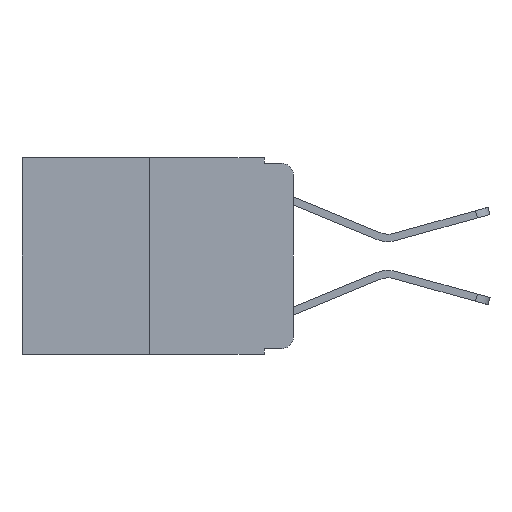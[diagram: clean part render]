
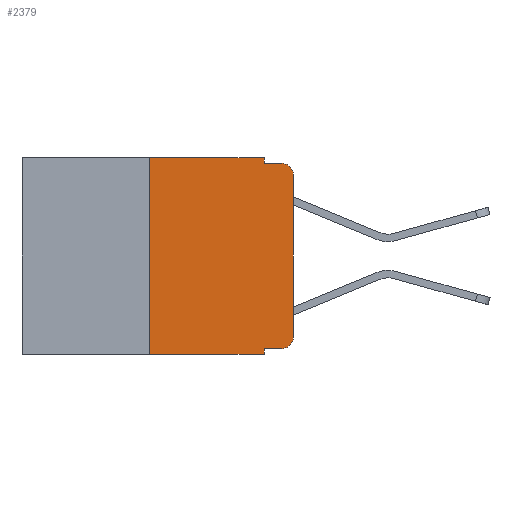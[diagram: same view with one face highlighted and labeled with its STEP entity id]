
A CAD part, left-side view. The second image highlights one B-rep face of the part: STEP entity #2379.
In plain terms, the highlighted planar face has unit normal (-1, 0, 0).
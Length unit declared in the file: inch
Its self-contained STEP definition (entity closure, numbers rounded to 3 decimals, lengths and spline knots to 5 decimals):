
#25 = CARTESIAN_POINT ( 'NONE',  ( 0., 0.473, -0.343 ) ) ;
#545 = EDGE_CURVE ( 'NONE', #8160, #2380, #8892, .T. ) ;
#1359 = ORIENTED_EDGE ( 'NONE', *, *, #10908, .F. ) ;
#1420 = DIRECTION ( 'NONE',  ( 0., -1., 0. ) ) ;
#1540 = CARTESIAN_POINT ( 'NONE',  ( 0., 0.02, -0.313 ) ) ;
#1792 = LINE ( 'NONE', #3881, #6658 ) ;
#1939 = ORIENTED_EDGE ( 'NONE', *, *, #9270, .T. ) ;
#1943 = CARTESIAN_POINT ( 'NONE',  ( 0., 0.051, -0.333 ) ) ;
#2121 = LINE ( 'NONE', #12446, #9585 ) ;
#2138 = CARTESIAN_POINT ( 'NONE',  ( 0., 0.02, -0.01 ) ) ;
#2359 = CARTESIAN_POINT ( 'NONE',  ( 0., 0.051, -0.333 ) ) ;
#2379 = ADVANCED_FACE ( 'NONE', ( #4698 ), #5224, .F. ) ;
#2380 = VERTEX_POINT ( 'NONE', #7279 ) ;
#2382 = DIRECTION ( 'NONE',  ( 0., 0., -1. ) ) ;
#2457 = DIRECTION ( 'NONE',  ( 0., 0., -1. ) ) ;
#2760 = EDGE_CURVE ( 'NONE', #7837, #12146, #2121, .T. ) ;
#2999 = LINE ( 'NONE', #8711, #10613 ) ;
#3155 = EDGE_CURVE ( 'NONE', #3417, #4068, #8963, .T. ) ;
#3320 = CARTESIAN_POINT ( 'NONE',  ( 0., 0.473, 0. ) ) ;
#3417 = VERTEX_POINT ( 'NONE', #5124 ) ;
#3602 = CARTESIAN_POINT ( 'NONE',  ( 0., 0.25, 0. ) ) ;
#3806 = CARTESIAN_POINT ( 'NONE',  ( 0., 0.02, -0.03 ) ) ;
#3844 = EDGE_CURVE ( 'NONE', #7837, #10011, #12469, .T. ) ;
#3881 = CARTESIAN_POINT ( 'NONE',  ( 0., 0., 0. ) ) ;
#4068 = VERTEX_POINT ( 'NONE', #2138 ) ;
#4151 = VECTOR ( 'NONE', #2457, 39.37008 ) ;
#4209 = ORIENTED_EDGE ( 'NONE', *, *, #10616, .T. ) ;
#4503 = DIRECTION ( 'NONE',  ( 0., 0., -1. ) ) ;
#4657 = EDGE_CURVE ( 'NONE', #2380, #4068, #2999, .T. ) ;
#4698 = FACE_OUTER_BOUND ( 'NONE', #8958, .T. ) ;
#4731 = DIRECTION ( 'NONE',  ( -1., 0., 0. ) ) ;
#4847 = CIRCLE ( 'NONE', #7038, 0.02 ) ;
#5124 = CARTESIAN_POINT ( 'NONE',  ( 0., 0., -0.03 ) ) ;
#5224 = PLANE ( 'NONE',  #9424 ) ;
#5274 = LINE ( 'NONE', #25, #11707 ) ;
#5377 = CARTESIAN_POINT ( 'NONE',  ( 0., 0.051, 0. ) ) ;
#5508 = ORIENTED_EDGE ( 'NONE', *, *, #545, .F. ) ;
#5880 = DIRECTION ( 'NONE',  ( 0., -1., 0. ) ) ;
#5904 = CARTESIAN_POINT ( 'NONE',  ( 0., 0.051, -0.343 ) ) ;
#6090 = CARTESIAN_POINT ( 'NONE',  ( 0., 0.473, 0. ) ) ;
#6315 = DIRECTION ( 'NONE',  ( 0., 0., 1. ) ) ;
#6441 = ORIENTED_EDGE ( 'NONE', *, *, #3155, .T. ) ;
#6626 = CARTESIAN_POINT ( 'NONE',  ( 0., 0.02, -0.333 ) ) ;
#6658 = VECTOR ( 'NONE', #9770, 39.37008 ) ;
#6775 = CARTESIAN_POINT ( 'NONE',  ( 0., 0.051, 0. ) ) ;
#6785 = ORIENTED_EDGE ( 'NONE', *, *, #8420, .F. ) ;
#7038 = AXIS2_PLACEMENT_3D ( 'NONE', #1540, #11309, #4503 ) ;
#7279 = CARTESIAN_POINT ( 'NONE',  ( 0., 0.051, -0.01 ) ) ;
#7557 = DIRECTION ( 'NONE',  ( 0., 0., -1. ) ) ;
#7759 = VERTEX_POINT ( 'NONE', #12002 ) ;
#7837 = VERTEX_POINT ( 'NONE', #2359 ) ;
#8046 = CARTESIAN_POINT ( 'NONE',  ( 0., 0.25, 0. ) ) ;
#8160 = VERTEX_POINT ( 'NONE', #6775 ) ;
#8383 = ORIENTED_EDGE ( 'NONE', *, *, #4657, .F. ) ;
#8420 = EDGE_CURVE ( 'NONE', #11962, #8160, #11314, .T. ) ;
#8455 = ORIENTED_EDGE ( 'NONE', *, *, #3844, .T. ) ;
#8711 = CARTESIAN_POINT ( 'NONE',  ( 0., 0.051, -0.01 ) ) ;
#8729 = DIRECTION ( 'NONE',  ( 0., -1., 0. ) ) ;
#8892 = LINE ( 'NONE', #5377, #4151 ) ;
#8958 = EDGE_LOOP ( 'NONE', ( #4209, #6441, #8383, #5508, #6785, #1359, #10293, #10185, #8455, #1939 ) ) ;
#8963 = CIRCLE ( 'NONE', #9103, 0.02 ) ;
#9088 = VERTEX_POINT ( 'NONE', #10236 ) ;
#9103 = AXIS2_PLACEMENT_3D ( 'NONE', #3806, #4731, #7557 ) ;
#9270 = EDGE_CURVE ( 'NONE', #10011, #7759, #4847, .T. ) ;
#9424 = AXIS2_PLACEMENT_3D ( 'NONE', #3320, #10134, #2382 ) ;
#9558 = LINE ( 'NONE', #8046, #10287 ) ;
#9585 = VECTOR ( 'NONE', #12534, 39.37008 ) ;
#9616 = DIRECTION ( 'NONE',  ( 0., -1., 0. ) ) ;
#9770 = DIRECTION ( 'NONE',  ( 0., 0., 1. ) ) ;
#10011 = VERTEX_POINT ( 'NONE', #6626 ) ;
#10075 = VECTOR ( 'NONE', #1420, 39.37008 ) ;
#10134 = DIRECTION ( 'NONE',  ( 1., 0., 0. ) ) ;
#10185 = ORIENTED_EDGE ( 'NONE', *, *, #2760, .F. ) ;
#10236 = CARTESIAN_POINT ( 'NONE',  ( 0., 0.25, -0.343 ) ) ;
#10287 = VECTOR ( 'NONE', #6315, 39.37008 ) ;
#10293 = ORIENTED_EDGE ( 'NONE', *, *, #11364, .T. ) ;
#10353 = VECTOR ( 'NONE', #5880, 39.37008 ) ;
#10613 = VECTOR ( 'NONE', #9616, 39.37008 ) ;
#10616 = EDGE_CURVE ( 'NONE', #7759, #3417, #1792, .T. ) ;
#10908 = EDGE_CURVE ( 'NONE', #9088, #11962, #9558, .T. ) ;
#11309 = DIRECTION ( 'NONE',  ( -1., 0., 0. ) ) ;
#11314 = LINE ( 'NONE', #6090, #10075 ) ;
#11364 = EDGE_CURVE ( 'NONE', #9088, #12146, #5274, .T. ) ;
#11707 = VECTOR ( 'NONE', #8729, 39.37008 ) ;
#11962 = VERTEX_POINT ( 'NONE', #3602 ) ;
#12002 = CARTESIAN_POINT ( 'NONE',  ( 0., 0., -0.313 ) ) ;
#12146 = VERTEX_POINT ( 'NONE', #5904 ) ;
#12446 = CARTESIAN_POINT ( 'NONE',  ( 0., 0.051, 0. ) ) ;
#12469 = LINE ( 'NONE', #1943, #10353 ) ;
#12534 = DIRECTION ( 'NONE',  ( 0., 0., -1. ) ) ;
